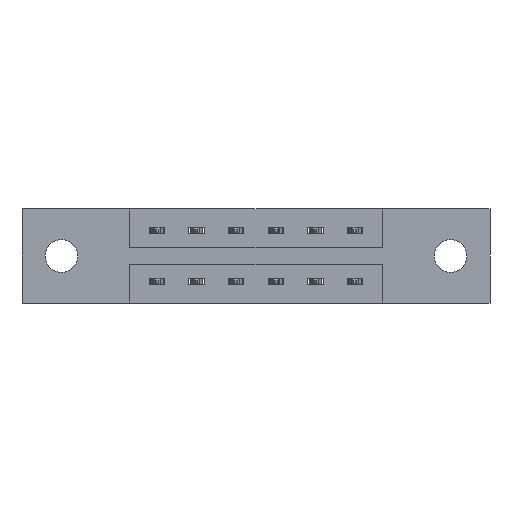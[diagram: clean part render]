
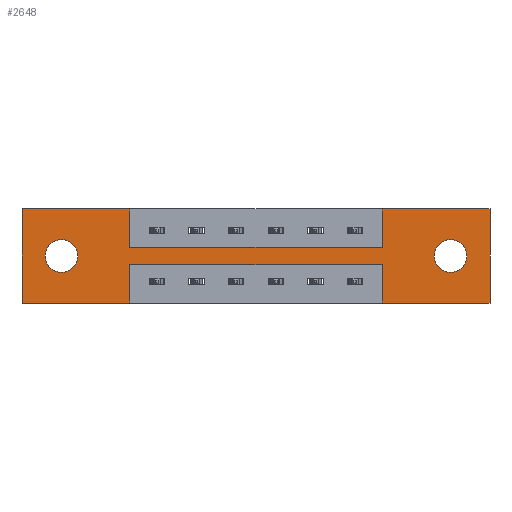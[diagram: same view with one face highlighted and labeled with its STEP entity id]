
A CAD part, front view. The second image highlights one B-rep face of the part: STEP entity #2648.
In plain terms, the highlighted planar face has unit normal (0, -1, 0).
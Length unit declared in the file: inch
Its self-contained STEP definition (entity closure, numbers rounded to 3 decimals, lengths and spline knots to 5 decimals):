
#95 = FACE_OUTER_BOUND ( 'NONE', #180, .T. ) ;
#109 = ORIENTED_EDGE ( 'NONE', *, *, #8280, .T. ) ;
#180 = EDGE_LOOP ( 'NONE', ( #2615, #7881, #1030, #7665, #1692, #7742, #5875, #812, #4336, #7141, #1955, #3115 ) ) ;
#212 = DIRECTION ( 'NONE',  ( -1., 0., 0. ) ) ;
#308 = VERTEX_POINT ( 'NONE', #4724 ) ;
#344 = FACE_BOUND ( 'NONE', #2187, .T. ) ;
#562 = VECTOR ( 'NONE', #8202, 39.37008 ) ;
#578 = AXIS2_PLACEMENT_3D ( 'NONE', #7870, #3697, #8555 ) ;
#636 = EDGE_CURVE ( 'NONE', #6168, #308, #7385, .T. ) ;
#784 = DIRECTION ( 'NONE',  ( 1., 0., 0. ) ) ;
#812 = ORIENTED_EDGE ( 'NONE', *, *, #6175, .F. ) ;
#845 = VERTEX_POINT ( 'NONE', #2994 ) ;
#876 = CARTESIAN_POINT ( 'NONE',  ( 0., 0., 0. ) ) ;
#1027 = PLANE ( 'NONE',  #2415 ) ;
#1030 = ORIENTED_EDGE ( 'NONE', *, *, #7116, .F. ) ;
#1082 = VERTEX_POINT ( 'NONE', #5741 ) ;
#1106 = DIRECTION ( 'NONE',  ( 0., 0., 1. ) ) ;
#1246 = CARTESIAN_POINT ( 'NONE',  ( 1.417, 0., -0.15 ) ) ;
#1293 = DIRECTION ( 'NONE',  ( 0., 0., 1. ) ) ;
#1306 = CIRCLE ( 'NONE', #4287, 0.064 ) ;
#1361 = VECTOR ( 'NONE', #3601, 39.37008 ) ;
#1426 = DIRECTION ( 'NONE',  ( 0., 1., 0. ) ) ;
#1433 = CARTESIAN_POINT ( 'NONE',  ( 0.155, 0., -0.185 ) ) ;
#1692 = ORIENTED_EDGE ( 'NONE', *, *, #636, .F. ) ;
#1955 = ORIENTED_EDGE ( 'NONE', *, *, #4650, .F. ) ;
#1965 = FACE_BOUND ( 'NONE', #3916, .T. ) ;
#2001 = LINE ( 'NONE', #9068, #5604 ) ;
#2086 = DIRECTION ( 'NONE',  ( 1., 0., 0. ) ) ;
#2145 = EDGE_CURVE ( 'NONE', #8629, #8668, #1306, .T. ) ;
#2187 = EDGE_LOOP ( 'NONE', ( #7656, #3941 ) ) ;
#2200 = VECTOR ( 'NONE', #5909, 39.37008 ) ;
#2237 = VERTEX_POINT ( 'NONE', #6628 ) ;
#2415 = AXIS2_PLACEMENT_3D ( 'NONE', #4139, #8033, #7884 ) ;
#2430 = AXIS2_PLACEMENT_3D ( 'NONE', #7001, #2817, #8323 ) ;
#2492 = CARTESIAN_POINT ( 'NONE',  ( 1.687, 0., -0.185 ) ) ;
#2508 = CARTESIAN_POINT ( 'NONE',  ( 1.417, 0., 0. ) ) ;
#2570 = DIRECTION ( 'NONE',  ( 0., 0., 1. ) ) ;
#2615 = ORIENTED_EDGE ( 'NONE', *, *, #8924, .F. ) ;
#2648 = ADVANCED_FACE ( 'NONE', ( #1965, #344, #95 ), #1027, .T. ) ;
#2750 = LINE ( 'NONE', #8662, #562 ) ;
#2817 = DIRECTION ( 'NONE',  ( 0., 1., 0. ) ) ;
#2994 = CARTESIAN_POINT ( 'NONE',  ( 1.417, 0., -0.22 ) ) ;
#3054 = EDGE_CURVE ( 'NONE', #3820, #1082, #2750, .T. ) ;
#3060 = VERTEX_POINT ( 'NONE', #2508 ) ;
#3115 = ORIENTED_EDGE ( 'NONE', *, *, #3054, .F. ) ;
#3124 = CARTESIAN_POINT ( 'NONE',  ( 0., 0., 0. ) ) ;
#3343 = CARTESIAN_POINT ( 'NONE',  ( 0., 0., 0. ) ) ;
#3404 = VECTOR ( 'NONE', #2086, 39.37008 ) ;
#3518 = LINE ( 'NONE', #3343, #1361 ) ;
#3601 = DIRECTION ( 'NONE',  ( 1., 0., 0. ) ) ;
#3697 = DIRECTION ( 'NONE',  ( 0., 1., 0. ) ) ;
#3820 = VERTEX_POINT ( 'NONE', #5939 ) ;
#3884 = EDGE_CURVE ( 'NONE', #6540, #4235, #7761, .T. ) ;
#3916 = EDGE_LOOP ( 'NONE', ( #6258, #109 ) ) ;
#3941 = ORIENTED_EDGE ( 'NONE', *, *, #3884, .T. ) ;
#3991 = LINE ( 'NONE', #6321, #8470 ) ;
#4044 = CARTESIAN_POINT ( 'NONE',  ( 0.155, 0., -0.249 ) ) ;
#4139 = CARTESIAN_POINT ( 'NONE',  ( 0., 0., -0.37 ) ) ;
#4209 = CARTESIAN_POINT ( 'NONE',  ( 1.842, 0., 0. ) ) ;
#4235 = VERTEX_POINT ( 'NONE', #4578 ) ;
#4287 = AXIS2_PLACEMENT_3D ( 'NONE', #2492, #7803, #7520 ) ;
#4336 = ORIENTED_EDGE ( 'NONE', *, *, #5678, .F. ) ;
#4363 = EDGE_CURVE ( 'NONE', #308, #6123, #5662, .T. ) ;
#4420 = VERTEX_POINT ( 'NONE', #7474 ) ;
#4578 = CARTESIAN_POINT ( 'NONE',  ( 0.155, 0., -0.121 ) ) ;
#4650 = EDGE_CURVE ( 'NONE', #1082, #5674, #9006, .T. ) ;
#4724 = CARTESIAN_POINT ( 'NONE',  ( 1.842, 0., -0.37 ) ) ;
#4871 = DIRECTION ( 'NONE',  ( -1., 0., 0. ) ) ;
#4901 = CARTESIAN_POINT ( 'NONE',  ( 0.425, 0., -0.15 ) ) ;
#4963 = LINE ( 'NONE', #876, #3404 ) ;
#5381 = DIRECTION ( 'NONE',  ( 0., 0., -1. ) ) ;
#5432 = VECTOR ( 'NONE', #4871, 39.37008 ) ;
#5497 = VECTOR ( 'NONE', #6497, 39.37008 ) ;
#5537 = VERTEX_POINT ( 'NONE', #1246 ) ;
#5604 = VECTOR ( 'NONE', #8409, 39.37008 ) ;
#5662 = LINE ( 'NONE', #7450, #5432 ) ;
#5674 = VERTEX_POINT ( 'NONE', #8441 ) ;
#5678 = EDGE_CURVE ( 'NONE', #4420, #2237, #8902, .T. ) ;
#5699 = EDGE_CURVE ( 'NONE', #5674, #4420, #4963, .T. ) ;
#5741 = CARTESIAN_POINT ( 'NONE',  ( 0., 0., -0.37 ) ) ;
#5875 = ORIENTED_EDGE ( 'NONE', *, *, #6643, .F. ) ;
#5909 = DIRECTION ( 'NONE',  ( 0., 0., 1. ) ) ;
#5939 = CARTESIAN_POINT ( 'NONE',  ( 0.425, 0., -0.37 ) ) ;
#6123 = VERTEX_POINT ( 'NONE', #6801 ) ;
#6168 = VERTEX_POINT ( 'NONE', #6809 ) ;
#6175 = EDGE_CURVE ( 'NONE', #2237, #5537, #7209, .T. ) ;
#6182 = EDGE_CURVE ( 'NONE', #3060, #6168, #3518, .T. ) ;
#6249 = CARTESIAN_POINT ( 'NONE',  ( 0.425, 0., 0. ) ) ;
#6258 = ORIENTED_EDGE ( 'NONE', *, *, #2145, .T. ) ;
#6321 = CARTESIAN_POINT ( 'NONE',  ( 1.417, 0., -0.37 ) ) ;
#6342 = VERTEX_POINT ( 'NONE', #7114 ) ;
#6412 = CARTESIAN_POINT ( 'NONE',  ( 1.687, 0., -0.121 ) ) ;
#6497 = DIRECTION ( 'NONE',  ( 0., 0., -1. ) ) ;
#6540 = VERTEX_POINT ( 'NONE', #4044 ) ;
#6628 = CARTESIAN_POINT ( 'NONE',  ( 0.425, 0., -0.15 ) ) ;
#6643 = EDGE_CURVE ( 'NONE', #5537, #3060, #7842, .T. ) ;
#6801 = CARTESIAN_POINT ( 'NONE',  ( 1.417, 0., -0.37 ) ) ;
#6809 = CARTESIAN_POINT ( 'NONE',  ( 1.842, 0., 0. ) ) ;
#6868 = VECTOR ( 'NONE', #5381, 39.37008 ) ;
#7001 = CARTESIAN_POINT ( 'NONE',  ( 1.687, 0., -0.185 ) ) ;
#7114 = CARTESIAN_POINT ( 'NONE',  ( 0.425, 0., -0.22 ) ) ;
#7116 = EDGE_CURVE ( 'NONE', #6123, #845, #3991, .T. ) ;
#7141 = ORIENTED_EDGE ( 'NONE', *, *, #5699, .F. ) ;
#7209 = LINE ( 'NONE', #4901, #8807 ) ;
#7385 = LINE ( 'NONE', #4209, #5497 ) ;
#7450 = CARTESIAN_POINT ( 'NONE',  ( 0., 0., -0.37 ) ) ;
#7451 = CARTESIAN_POINT ( 'NONE',  ( 0.425, 0., -0.22 ) ) ;
#7474 = CARTESIAN_POINT ( 'NONE',  ( 0.425, 0., 0. ) ) ;
#7520 = DIRECTION ( 'NONE',  ( 0., 0., -1. ) ) ;
#7574 = EDGE_CURVE ( 'NONE', #845, #6342, #9267, .T. ) ;
#7597 = CIRCLE ( 'NONE', #578, 0.064 ) ;
#7628 = VECTOR ( 'NONE', #1106, 39.37008 ) ;
#7656 = ORIENTED_EDGE ( 'NONE', *, *, #9343, .T. ) ;
#7665 = ORIENTED_EDGE ( 'NONE', *, *, #4363, .F. ) ;
#7682 = AXIS2_PLACEMENT_3D ( 'NONE', #1433, #1426, #1293 ) ;
#7742 = ORIENTED_EDGE ( 'NONE', *, *, #6182, .F. ) ;
#7761 = CIRCLE ( 'NONE', #7682, 0.064 ) ;
#7803 = DIRECTION ( 'NONE',  ( 0., 1., 0. ) ) ;
#7842 = LINE ( 'NONE', #8653, #7628 ) ;
#7870 = CARTESIAN_POINT ( 'NONE',  ( 0.155, 0., -0.185 ) ) ;
#7881 = ORIENTED_EDGE ( 'NONE', *, *, #7574, .F. ) ;
#7884 = DIRECTION ( 'NONE',  ( 0., 0., -1. ) ) ;
#7940 = CIRCLE ( 'NONE', #2430, 0.064 ) ;
#8033 = DIRECTION ( 'NONE',  ( 0., -1., 0. ) ) ;
#8202 = DIRECTION ( 'NONE',  ( -1., 0., 0. ) ) ;
#8280 = EDGE_CURVE ( 'NONE', #8668, #8629, #7940, .T. ) ;
#8323 = DIRECTION ( 'NONE',  ( 0., 0., -1. ) ) ;
#8409 = DIRECTION ( 'NONE',  ( 0., 0., -1. ) ) ;
#8441 = CARTESIAN_POINT ( 'NONE',  ( 0., 0., 0. ) ) ;
#8470 = VECTOR ( 'NONE', #2570, 39.37008 ) ;
#8555 = DIRECTION ( 'NONE',  ( 0., 0., 1. ) ) ;
#8629 = VERTEX_POINT ( 'NONE', #6412 ) ;
#8653 = CARTESIAN_POINT ( 'NONE',  ( 1.417, 0., 0. ) ) ;
#8662 = CARTESIAN_POINT ( 'NONE',  ( 0., 0., -0.37 ) ) ;
#8668 = VERTEX_POINT ( 'NONE', #9291 ) ;
#8807 = VECTOR ( 'NONE', #784, 39.37008 ) ;
#8902 = LINE ( 'NONE', #6249, #6868 ) ;
#8924 = EDGE_CURVE ( 'NONE', #6342, #3820, #2001, .T. ) ;
#9006 = LINE ( 'NONE', #3124, #2200 ) ;
#9068 = CARTESIAN_POINT ( 'NONE',  ( 0.425, 0., -0.37 ) ) ;
#9087 = VECTOR ( 'NONE', #212, 39.37008 ) ;
#9267 = LINE ( 'NONE', #7451, #9087 ) ;
#9291 = CARTESIAN_POINT ( 'NONE',  ( 1.687, 0., -0.249 ) ) ;
#9343 = EDGE_CURVE ( 'NONE', #4235, #6540, #7597, .T. ) ;
